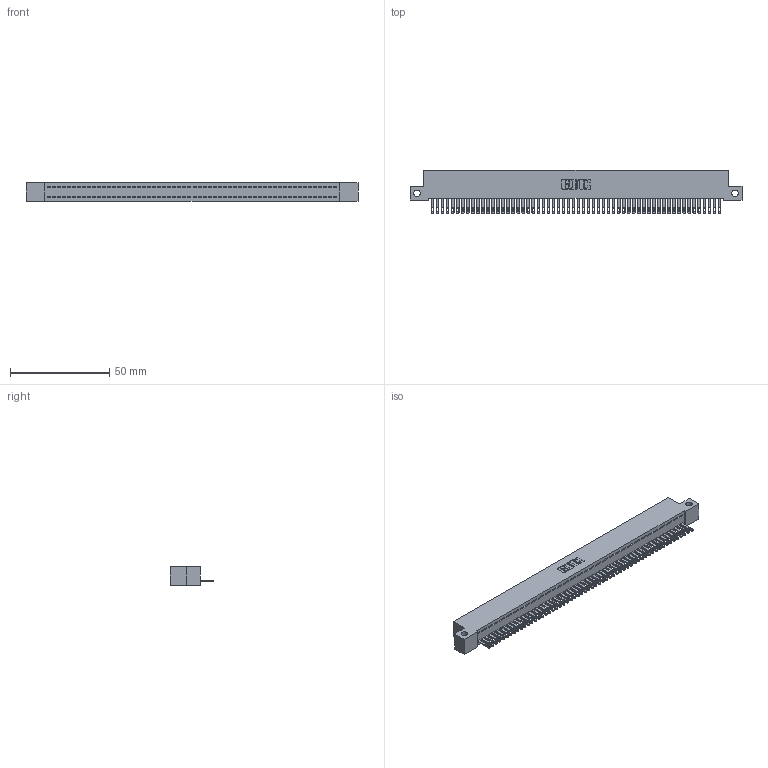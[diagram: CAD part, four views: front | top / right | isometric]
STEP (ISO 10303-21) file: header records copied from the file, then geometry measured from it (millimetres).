
FILE_DESCRIPTION (( 'STEP AP203' ), '1' );
FILE_NAME ('342-058-500-112.STEP', '2018-08-13T04:48:49', ( '' ), ( '' ), 'SwSTEP 2.0', 'SolidWorks 2016', '' );
FILE_SCHEMA (( 'CONFIG_CONTROL_DESIGN' ));
Length unit declared in the file: inch
Products named in the file (3): 342 Part_Side Mount; 345-292-001_345-293-100; 342-058-500-112
Assembly tree (59 placements, depth 2):
  342-058-500-112
    342 Part_Side Mount
    345-292-001_345-293-100  x58
Bounding box: 167.64 x 21.85 x 9.4 mm (x, y, z)
Volume: 14719.6 mm3; surface area: 21864.9 mm2
Topology: 59 solids, 59 shells, 3242 faces, 10043 edges, 6694 vertices
Faces by surface type: plane 2154, cylinder 1088
Entity records: 33189 total; most frequent: CARTESIAN_POINT 5728, ORIENTED_EDGE 5722, DIRECTION 4801, EDGE_CURVE 2861, VECTOR 2729, LINE 2729, VERTEX_POINT 1906, AXIS2_PLACEMENT_3D 1036
